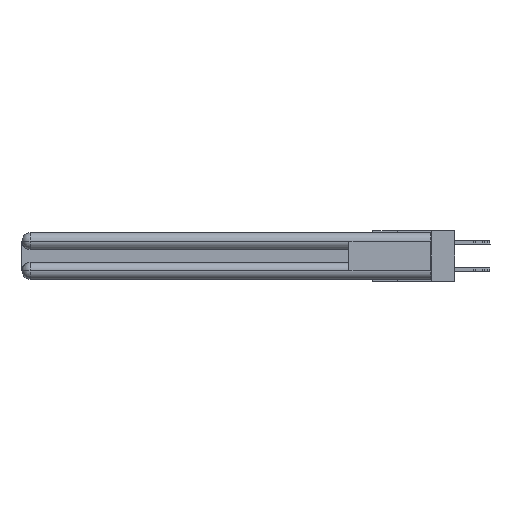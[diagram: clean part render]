
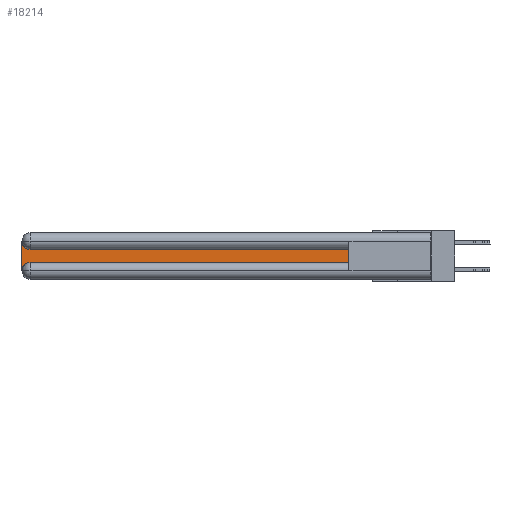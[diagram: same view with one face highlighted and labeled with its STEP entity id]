
A CAD part, left-side view. The second image highlights one B-rep face of the part: STEP entity #18214.
In plain terms, the highlighted planar face has unit normal (-1, 0, 0).
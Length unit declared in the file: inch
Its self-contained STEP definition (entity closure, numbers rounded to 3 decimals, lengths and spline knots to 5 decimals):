
#496 = VERTEX_POINT ( 'NONE', #29493 ) ;
#1134 = LINE ( 'NONE', #4413, #14049 ) ;
#1529 = CARTESIAN_POINT ( 'NONE',  ( 0.075, 2.94, -0.2175 ) ) ;
#1777 = CARTESIAN_POINT ( 'NONE',  ( 0.075, 3., -0.1225 ) ) ;
#2166 = EDGE_CURVE ( 'NONE', #24043, #496, #11739, .T. ) ;
#2412 = CARTESIAN_POINT ( 'NONE',  ( 0.075, 0.6, -0.2175 ) ) ;
#3348 = VERTEX_POINT ( 'NONE', #4142 ) ;
#4142 = CARTESIAN_POINT ( 'NONE',  ( 0.075, 3., -0.2775 ) ) ;
#4413 = CARTESIAN_POINT ( 'NONE',  ( 0.075, 0.6, -0.2175 ) ) ;
#4771 = CARTESIAN_POINT ( 'NONE',  ( 0.075, 0.6, -0.2175 ) ) ;
#4789 = VERTEX_POINT ( 'NONE', #1529 ) ;
#4985 = CARTESIAN_POINT ( 'NONE',  ( 0.075, 2.94, -0.0625 ) ) ;
#5945 = EDGE_CURVE ( 'NONE', #8968, #9228, #23719, .T. ) ;
#6989 = PLANE ( 'NONE',  #23786 ) ;
#7461 = EDGE_CURVE ( 'NONE', #3348, #4789, #32086, .T. ) ;
#8089 = EDGE_LOOP ( 'NONE', ( #16402, #10816, #26157, #33268, #13516, #19173 ) ) ;
#8968 = VERTEX_POINT ( 'NONE', #22509 ) ;
#9228 = VERTEX_POINT ( 'NONE', #30823 ) ;
#9960 = EDGE_CURVE ( 'NONE', #4789, #24043, #1134, .T. ) ;
#10180 = DIRECTION ( 'NONE',  ( 0., 0., 1. ) ) ;
#10816 = ORIENTED_EDGE ( 'NONE', *, *, #5945, .T. ) ;
#11739 = LINE ( 'NONE', #4771, #17373 ) ;
#12489 = LINE ( 'NONE', #24858, #14919 ) ;
#13516 = ORIENTED_EDGE ( 'NONE', *, *, #9960, .T. ) ;
#14049 = VECTOR ( 'NONE', #14445, 39.37008 ) ;
#14445 = DIRECTION ( 'NONE',  ( 0., -1., 0. ) ) ;
#14919 = VECTOR ( 'NONE', #19676, 39.37008 ) ;
#16402 = ORIENTED_EDGE ( 'NONE', *, *, #24761, .T. ) ;
#17373 = VECTOR ( 'NONE', #10180, 39.37008 ) ;
#17797 = VECTOR ( 'NONE', #32697, 39.37008 ) ;
#18214 = ADVANCED_FACE ( 'NONE', ( #26700 ), #6989, .F. ) ;
#19173 = ORIENTED_EDGE ( 'NONE', *, *, #2166, .T. ) ;
#19676 = DIRECTION ( 'NONE',  ( 0., 1., 0. ) ) ;
#22509 = CARTESIAN_POINT ( 'NONE',  ( 0.075, 2.94, -0.1225 ) ) ;
#22928 = DIRECTION ( 'NONE',  ( 1., 0., 0. ) ) ;
#23140 = CARTESIAN_POINT ( 'NONE',  ( 0.075, 2.94, -0.2775 ) ) ;
#23719 = CIRCLE ( 'NONE', #32617, 0.06 ) ;
#23786 = AXIS2_PLACEMENT_3D ( 'NONE', #1777, #29721, #32651 ) ;
#23956 = EDGE_CURVE ( 'NONE', #9228, #3348, #30261, .T. ) ;
#24043 = VERTEX_POINT ( 'NONE', #2412 ) ;
#24761 = EDGE_CURVE ( 'NONE', #496, #8968, #12489, .T. ) ;
#24858 = CARTESIAN_POINT ( 'NONE',  ( 0.075, 0.6, -0.1225 ) ) ;
#25467 = DIRECTION ( 'NONE',  ( 0., 0., -1. ) ) ;
#26157 = ORIENTED_EDGE ( 'NONE', *, *, #23956, .T. ) ;
#26700 = FACE_OUTER_BOUND ( 'NONE', #8089, .T. ) ;
#28295 = DIRECTION ( 'NONE',  ( 1., 0., 0. ) ) ;
#29493 = CARTESIAN_POINT ( 'NONE',  ( 0.075, 0.6, -0.1225 ) ) ;
#29721 = DIRECTION ( 'NONE',  ( 1., 0., 0. ) ) ;
#30261 = LINE ( 'NONE', #32482, #17797 ) ;
#30692 = DIRECTION ( 'NONE',  ( 0., 0., -1. ) ) ;
#30823 = CARTESIAN_POINT ( 'NONE',  ( 0.075, 3., -0.0625 ) ) ;
#31313 = AXIS2_PLACEMENT_3D ( 'NONE', #23140, #22928, #30692 ) ;
#32086 = CIRCLE ( 'NONE', #31313, 0.06 ) ;
#32482 = CARTESIAN_POINT ( 'NONE',  ( 0.075, 3., -0.2175 ) ) ;
#32617 = AXIS2_PLACEMENT_3D ( 'NONE', #4985, #28295, #25467 ) ;
#32651 = DIRECTION ( 'NONE',  ( 0., 0., -1. ) ) ;
#32697 = DIRECTION ( 'NONE',  ( 0., 0., -1. ) ) ;
#33268 = ORIENTED_EDGE ( 'NONE', *, *, #7461, .T. ) ;
